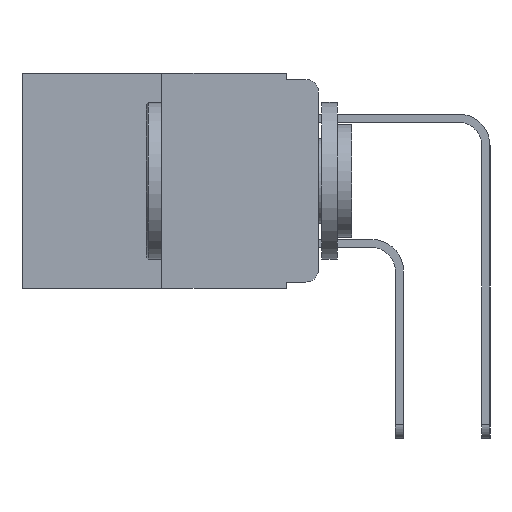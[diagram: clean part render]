
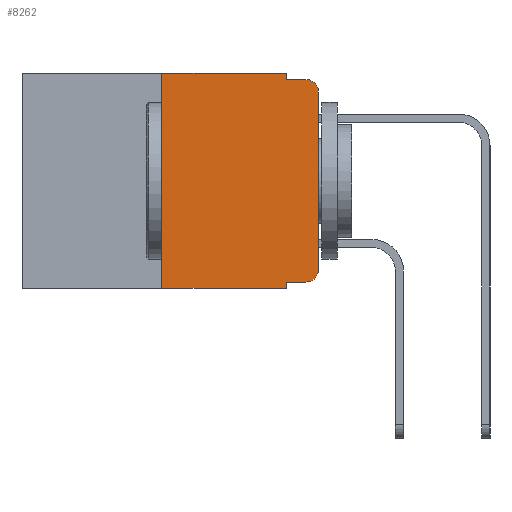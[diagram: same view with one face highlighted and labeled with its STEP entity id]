
A CAD part, left-side view. The second image highlights one B-rep face of the part: STEP entity #8262.
In plain terms, the highlighted planar face has unit normal (-1, 0, 0).
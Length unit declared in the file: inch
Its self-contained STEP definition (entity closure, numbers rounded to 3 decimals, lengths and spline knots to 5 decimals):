
#9 = ORIENTED_EDGE ( 'NONE', *, *, #11235, .T. ) ;
#314 = CARTESIAN_POINT ( 'NONE',  ( 0., 0.02, -0.333 ) ) ;
#362 = EDGE_CURVE ( 'NONE', #12396, #13585, #3896, .T. ) ;
#823 = CARTESIAN_POINT ( 'NONE',  ( 0., 0.473, 0. ) ) ;
#1225 = LINE ( 'NONE', #5045, #1618 ) ;
#1405 = DIRECTION ( 'NONE',  ( -1., 0., 0. ) ) ;
#1510 = CARTESIAN_POINT ( 'NONE',  ( 0., 0., -0.03 ) ) ;
#1618 = VECTOR ( 'NONE', #13981, 39.37008 ) ;
#1760 = VECTOR ( 'NONE', #4535, 39.37008 ) ;
#2009 = CIRCLE ( 'NONE', #6653, 0.02 ) ;
#2040 = CARTESIAN_POINT ( 'NONE',  ( 0., 0.051, 0. ) ) ;
#2098 = DIRECTION ( 'NONE',  ( 0., 0., -1. ) ) ;
#2167 = EDGE_CURVE ( 'NONE', #7686, #8820, #8381, .T. ) ;
#2417 = ORIENTED_EDGE ( 'NONE', *, *, #14045, .T. ) ;
#2755 = LINE ( 'NONE', #10252, #9179 ) ;
#3198 = LINE ( 'NONE', #8043, #12559 ) ;
#3211 = CARTESIAN_POINT ( 'NONE',  ( 0., 0.02, -0.03 ) ) ;
#3267 = ORIENTED_EDGE ( 'NONE', *, *, #9056, .T. ) ;
#3557 = VERTEX_POINT ( 'NONE', #11632 ) ;
#3896 = LINE ( 'NONE', #2040, #14082 ) ;
#4057 = ORIENTED_EDGE ( 'NONE', *, *, #362, .F. ) ;
#4107 = AXIS2_PLACEMENT_3D ( 'NONE', #3211, #12100, #4477 ) ;
#4158 = DIRECTION ( 'NONE',  ( 0., -1., 0. ) ) ;
#4306 = CARTESIAN_POINT ( 'NONE',  ( 0., 0.473, 0. ) ) ;
#4477 = DIRECTION ( 'NONE',  ( 0., 0., -1. ) ) ;
#4530 = VECTOR ( 'NONE', #4158, 39.37008 ) ;
#4535 = DIRECTION ( 'NONE',  ( 0., 0., -1. ) ) ;
#4937 = ORIENTED_EDGE ( 'NONE', *, *, #12507, .T. ) ;
#5045 = CARTESIAN_POINT ( 'NONE',  ( 0., 0.051, -0.333 ) ) ;
#5769 = CARTESIAN_POINT ( 'NONE',  ( 0., 0.051, 0. ) ) ;
#6555 = CARTESIAN_POINT ( 'NONE',  ( 0., 0., 0. ) ) ;
#6653 = AXIS2_PLACEMENT_3D ( 'NONE', #9064, #1405, #10308 ) ;
#6906 = ORIENTED_EDGE ( 'NONE', *, *, #13567, .F. ) ;
#7192 = PLANE ( 'NONE',  #11175 ) ;
#7686 = VERTEX_POINT ( 'NONE', #13685 ) ;
#8043 = CARTESIAN_POINT ( 'NONE',  ( 0., 0.25, 0. ) ) ;
#8165 = VERTEX_POINT ( 'NONE', #10763 ) ;
#8262 = ADVANCED_FACE ( 'NONE', ( #12370 ), #7192, .F. ) ;
#8308 = ORIENTED_EDGE ( 'NONE', *, *, #14261, .F. ) ;
#8381 = LINE ( 'NONE', #4306, #4530 ) ;
#8820 = VERTEX_POINT ( 'NONE', #14666 ) ;
#9056 = EDGE_CURVE ( 'NONE', #12396, #13544, #1225, .T. ) ;
#9064 = CARTESIAN_POINT ( 'NONE',  ( 0., 0.02, -0.313 ) ) ;
#9131 = DIRECTION ( 'NONE',  ( 0., 0., 1. ) ) ;
#9179 = VECTOR ( 'NONE', #14083, 39.37008 ) ;
#9309 = DIRECTION ( 'NONE',  ( 0., 0., 1. ) ) ;
#9404 = VERTEX_POINT ( 'NONE', #9512 ) ;
#9512 = CARTESIAN_POINT ( 'NONE',  ( 0., 0.25, -0.343 ) ) ;
#9748 = DIRECTION ( 'NONE',  ( 1., 0., 0. ) ) ;
#10252 = CARTESIAN_POINT ( 'NONE',  ( 0., 0.473, -0.343 ) ) ;
#10308 = DIRECTION ( 'NONE',  ( 0., 0., -1. ) ) ;
#10763 = CARTESIAN_POINT ( 'NONE',  ( 0., 0.051, -0.01 ) ) ;
#10807 = ORIENTED_EDGE ( 'NONE', *, *, #11256, .F. ) ;
#10996 = EDGE_CURVE ( 'NONE', #9404, #13585, #2755, .T. ) ;
#11175 = AXIS2_PLACEMENT_3D ( 'NONE', #823, #9748, #2098 ) ;
#11235 = EDGE_CURVE ( 'NONE', #14124, #15371, #16100, .T. ) ;
#11256 = EDGE_CURVE ( 'NONE', #8820, #8165, #12287, .T. ) ;
#11303 = EDGE_LOOP ( 'NONE', ( #4937, #9, #8308, #10807, #13666, #6906, #13056, #4057, #3267, #2417 ) ) ;
#11632 = CARTESIAN_POINT ( 'NONE',  ( 0., 0., -0.313 ) ) ;
#11788 = CARTESIAN_POINT ( 'NONE',  ( 0., 0.051, -0.343 ) ) ;
#12100 = DIRECTION ( 'NONE',  ( -1., 0., 0. ) ) ;
#12287 = LINE ( 'NONE', #5769, #1760 ) ;
#12370 = FACE_OUTER_BOUND ( 'NONE', #11303, .T. ) ;
#12396 = VERTEX_POINT ( 'NONE', #15243 ) ;
#12507 = EDGE_CURVE ( 'NONE', #3557, #14124, #16049, .T. ) ;
#12559 = VECTOR ( 'NONE', #9309, 39.37008 ) ;
#13056 = ORIENTED_EDGE ( 'NONE', *, *, #10996, .T. ) ;
#13544 = VERTEX_POINT ( 'NONE', #314 ) ;
#13567 = EDGE_CURVE ( 'NONE', #9404, #7686, #3198, .T. ) ;
#13585 = VERTEX_POINT ( 'NONE', #11788 ) ;
#13666 = ORIENTED_EDGE ( 'NONE', *, *, #2167, .F. ) ;
#13685 = CARTESIAN_POINT ( 'NONE',  ( 0., 0.25, 0. ) ) ;
#13748 = DIRECTION ( 'NONE',  ( 0., 0., -1. ) ) ;
#13981 = DIRECTION ( 'NONE',  ( 0., -1., 0. ) ) ;
#14045 = EDGE_CURVE ( 'NONE', #13544, #3557, #2009, .T. ) ;
#14082 = VECTOR ( 'NONE', #13748, 39.37008 ) ;
#14083 = DIRECTION ( 'NONE',  ( 0., -1., 0. ) ) ;
#14124 = VERTEX_POINT ( 'NONE', #1510 ) ;
#14261 = EDGE_CURVE ( 'NONE', #8165, #15371, #15360, .T. ) ;
#14341 = CARTESIAN_POINT ( 'NONE',  ( 0., 0.02, -0.01 ) ) ;
#14487 = CARTESIAN_POINT ( 'NONE',  ( 0., 0.051, -0.01 ) ) ;
#14666 = CARTESIAN_POINT ( 'NONE',  ( 0., 0.051, 0. ) ) ;
#14973 = VECTOR ( 'NONE', #15759, 39.37008 ) ;
#15243 = CARTESIAN_POINT ( 'NONE',  ( 0., 0.051, -0.333 ) ) ;
#15360 = LINE ( 'NONE', #14487, #14973 ) ;
#15371 = VERTEX_POINT ( 'NONE', #14341 ) ;
#15759 = DIRECTION ( 'NONE',  ( 0., -1., 0. ) ) ;
#16049 = LINE ( 'NONE', #6555, #16444 ) ;
#16100 = CIRCLE ( 'NONE', #4107, 0.02 ) ;
#16444 = VECTOR ( 'NONE', #9131, 39.37008 ) ;
